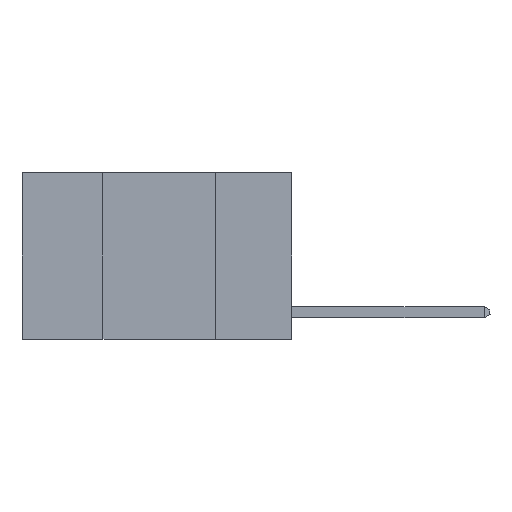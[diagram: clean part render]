
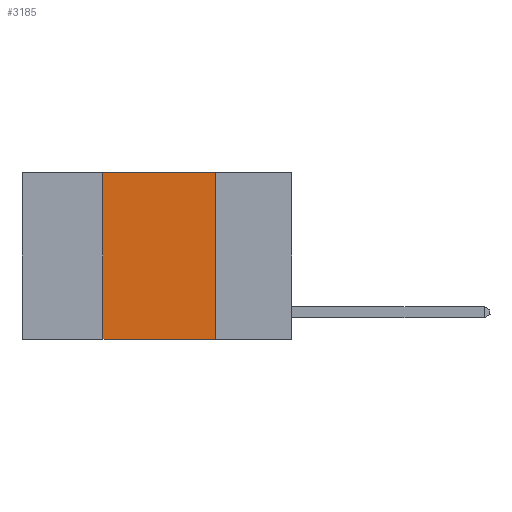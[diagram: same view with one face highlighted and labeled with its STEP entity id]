
A CAD part, left-side view. The second image highlights one B-rep face of the part: STEP entity #3185.
In plain terms, the highlighted planar face has unit normal (-1, 0, 0).
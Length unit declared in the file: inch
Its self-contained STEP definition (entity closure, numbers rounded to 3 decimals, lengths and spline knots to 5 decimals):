
#245 = LINE ( 'NONE', #5137, #1375 ) ;
#439 = ORIENTED_EDGE ( 'NONE', *, *, #2402, .F. ) ;
#585 = VERTEX_POINT ( 'NONE', #7368 ) ;
#778 = EDGE_CURVE ( 'NONE', #2602, #6885, #2502, .T. ) ;
#1170 = DIRECTION ( 'NONE',  ( 1., 0., 0. ) ) ;
#1375 = VECTOR ( 'NONE', #4426, 39.37008 ) ;
#1856 = FACE_OUTER_BOUND ( 'NONE', #6797, .T. ) ;
#2066 = CARTESIAN_POINT ( 'NONE',  ( 0., 0.6, 0. ) ) ;
#2174 = DIRECTION ( 'NONE',  ( 0., 0., -1. ) ) ;
#2402 = EDGE_CURVE ( 'NONE', #6885, #585, #3456, .T. ) ;
#2502 = LINE ( 'NONE', #5871, #5454 ) ;
#2602 = VERTEX_POINT ( 'NONE', #2679 ) ;
#2679 = CARTESIAN_POINT ( 'NONE',  ( 0., 0.42, 0. ) ) ;
#3185 = ADVANCED_FACE ( 'NONE', ( #1856 ), #5437, .F. ) ;
#3239 = VECTOR ( 'NONE', #7348, 39.37008 ) ;
#3456 = LINE ( 'NONE', #5955, #6185 ) ;
#4426 = DIRECTION ( 'NONE',  ( 0., -1., 0. ) ) ;
#4864 = DIRECTION ( 'NONE',  ( 0., 0., -1. ) ) ;
#5137 = CARTESIAN_POINT ( 'NONE',  ( 0., 0.6, -0.37 ) ) ;
#5437 = PLANE ( 'NONE',  #7710 ) ;
#5454 = VECTOR ( 'NONE', #9063, 39.37008 ) ;
#5871 = CARTESIAN_POINT ( 'NONE',  ( 0., 0.6, 0. ) ) ;
#5955 = CARTESIAN_POINT ( 'NONE',  ( 0., 0.17, 0. ) ) ;
#6185 = VECTOR ( 'NONE', #4864, 39.37008 ) ;
#6797 = EDGE_LOOP ( 'NONE', ( #439, #10204, #9833, #7497 ) ) ;
#6885 = VERTEX_POINT ( 'NONE', #6993 ) ;
#6993 = CARTESIAN_POINT ( 'NONE',  ( 0., 0.17, 0. ) ) ;
#7254 = LINE ( 'NONE', #8066, #3239 ) ;
#7348 = DIRECTION ( 'NONE',  ( 0., 0., 1. ) ) ;
#7368 = CARTESIAN_POINT ( 'NONE',  ( 0., 0.17, -0.37 ) ) ;
#7497 = ORIENTED_EDGE ( 'NONE', *, *, #9207, .T. ) ;
#7710 = AXIS2_PLACEMENT_3D ( 'NONE', #2066, #1170, #2174 ) ;
#8066 = CARTESIAN_POINT ( 'NONE',  ( 0., 0.42, 0. ) ) ;
#8537 = CARTESIAN_POINT ( 'NONE',  ( 0., 0.42, -0.37 ) ) ;
#9063 = DIRECTION ( 'NONE',  ( 0., -1., 0. ) ) ;
#9207 = EDGE_CURVE ( 'NONE', #9643, #585, #245, .T. ) ;
#9643 = VERTEX_POINT ( 'NONE', #8537 ) ;
#9741 = EDGE_CURVE ( 'NONE', #9643, #2602, #7254, .T. ) ;
#9833 = ORIENTED_EDGE ( 'NONE', *, *, #9741, .F. ) ;
#10204 = ORIENTED_EDGE ( 'NONE', *, *, #778, .F. ) ;
